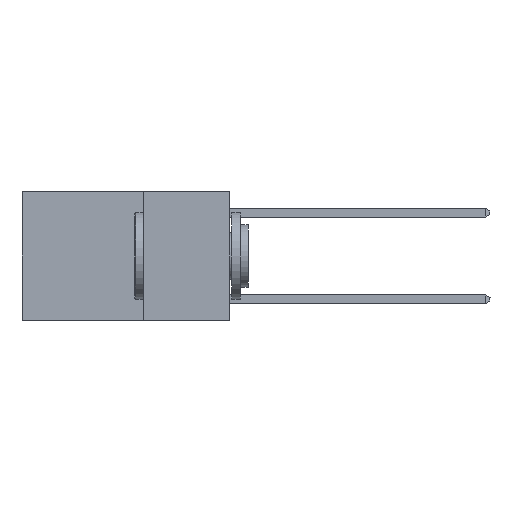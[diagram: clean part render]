
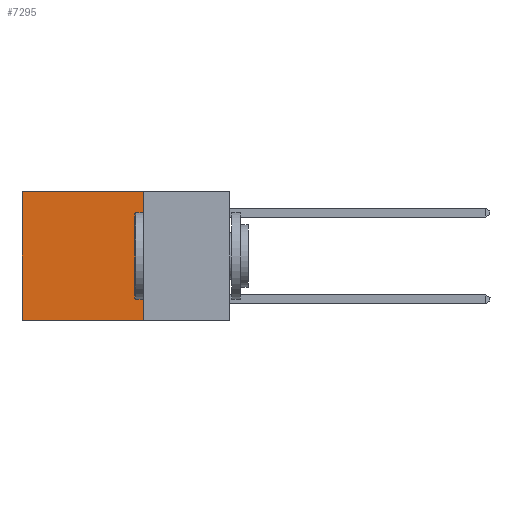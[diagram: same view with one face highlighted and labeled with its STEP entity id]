
A CAD part, left-side view. The second image highlights one B-rep face of the part: STEP entity #7295.
In plain terms, the highlighted planar face has unit normal (-1, 0, 0).
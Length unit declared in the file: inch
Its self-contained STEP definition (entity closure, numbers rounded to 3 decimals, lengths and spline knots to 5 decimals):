
#137 = DIRECTION ( 'NONE',  ( 1., 0., 0. ) ) ;
#1471 = CARTESIAN_POINT ( 'NONE',  ( 0.2625, 0.25, -0.37 ) ) ;
#2004 = EDGE_CURVE ( 'NONE', #16829, #19786, #12526, .T. ) ;
#2007 = VECTOR ( 'NONE', #7363, 39.37008 ) ;
#5137 = LINE ( 'NONE', #14750, #24919 ) ;
#5967 = DIRECTION ( 'NONE',  ( 0., 1., 0. ) ) ;
#7189 = DIRECTION ( 'NONE',  ( 0., 0., -1. ) ) ;
#7295 = ADVANCED_FACE ( 'NONE', ( #13996 ), #16187, .F. ) ;
#7363 = DIRECTION ( 'NONE',  ( 0., 1., 0. ) ) ;
#7367 = EDGE_CURVE ( 'NONE', #21568, #12991, #5137, .T. ) ;
#7503 = CARTESIAN_POINT ( 'NONE',  ( 0.2625, 0.25, 0. ) ) ;
#7885 = ORIENTED_EDGE ( 'NONE', *, *, #7367, .T. ) ;
#7896 = LINE ( 'NONE', #25165, #24570 ) ;
#8092 = CARTESIAN_POINT ( 'NONE',  ( 0.2625, 0.6, 0. ) ) ;
#10365 = CARTESIAN_POINT ( 'NONE',  ( 0.2625, 0.25, 0. ) ) ;
#11115 = VECTOR ( 'NONE', #22253, 39.37008 ) ;
#11227 = LINE ( 'NONE', #1471, #2007 ) ;
#12526 = LINE ( 'NONE', #10365, #11115 ) ;
#12991 = VERTEX_POINT ( 'NONE', #13826 ) ;
#13826 = CARTESIAN_POINT ( 'NONE',  ( 0.2625, 0.6, -0.37 ) ) ;
#13969 = ORIENTED_EDGE ( 'NONE', *, *, #20985, .F. ) ;
#13996 = FACE_OUTER_BOUND ( 'NONE', #17798, .T. ) ;
#14750 = CARTESIAN_POINT ( 'NONE',  ( 0.2625, 0.6, 0. ) ) ;
#16187 = PLANE ( 'NONE',  #16259 ) ;
#16259 = AXIS2_PLACEMENT_3D ( 'NONE', #22179, #137, #23962 ) ;
#16829 = VERTEX_POINT ( 'NONE', #7503 ) ;
#17798 = EDGE_LOOP ( 'NONE', ( #7885, #13969, #20310, #18042 ) ) ;
#18042 = ORIENTED_EDGE ( 'NONE', *, *, #18070, .T. ) ;
#18070 = EDGE_CURVE ( 'NONE', #16829, #21568, #7896, .T. ) ;
#19786 = VERTEX_POINT ( 'NONE', #21553 ) ;
#20310 = ORIENTED_EDGE ( 'NONE', *, *, #2004, .F. ) ;
#20985 = EDGE_CURVE ( 'NONE', #19786, #12991, #11227, .T. ) ;
#21553 = CARTESIAN_POINT ( 'NONE',  ( 0.2625, 0.25, -0.37 ) ) ;
#21568 = VERTEX_POINT ( 'NONE', #8092 ) ;
#22179 = CARTESIAN_POINT ( 'NONE',  ( 0.2625, 0.25, 0. ) ) ;
#22253 = DIRECTION ( 'NONE',  ( 0., 0., -1. ) ) ;
#23962 = DIRECTION ( 'NONE',  ( 0., 0., -1. ) ) ;
#24570 = VECTOR ( 'NONE', #5967, 39.37008 ) ;
#24919 = VECTOR ( 'NONE', #7189, 39.37008 ) ;
#25165 = CARTESIAN_POINT ( 'NONE',  ( 0.2625, 0.25, 0. ) ) ;
